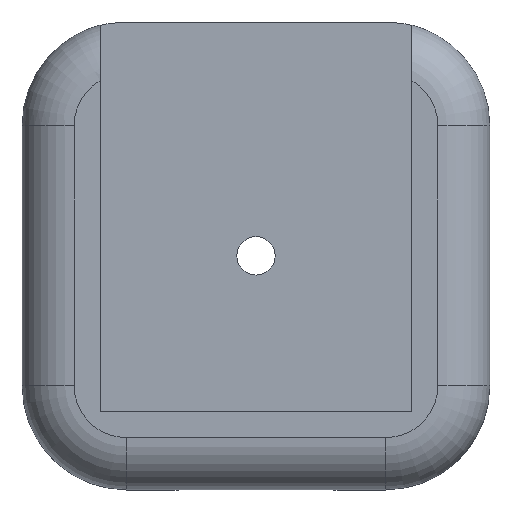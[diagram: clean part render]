
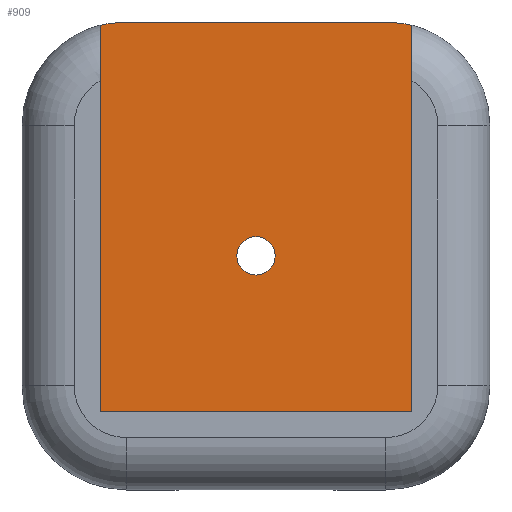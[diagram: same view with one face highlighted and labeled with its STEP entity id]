
A CAD part, top view. The second image highlights one B-rep face of the part: STEP entity #909.
In plain terms, the highlighted planar face has unit normal (0, 0, 1).
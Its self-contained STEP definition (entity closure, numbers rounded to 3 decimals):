
#11 = EDGE_CURVE ( 'NONE', #302, #878, #1433, .T. ) ;
#15 = AXIS2_PLACEMENT_3D ( 'NONE', #703, #1767, #857 ) ;
#23 = FACE_BOUND ( 'NONE', #1755, .T. ) ;
#51 = CIRCLE ( 'NONE', #916, 10. ) ;
#57 = AXIS2_PLACEMENT_3D ( 'NONE', #487, #1550, #638 ) ;
#63 = ORIENTED_EDGE ( 'NONE', *, *, #121, .T. ) ;
#78 = CIRCLE ( 'NONE', #57, 10. ) ;
#82 = ORIENTED_EDGE ( 'NONE', *, *, #1862, .T. ) ;
#83 = CIRCLE ( 'NONE', #15, 1.844 ) ;
#121 = EDGE_CURVE ( 'NONE', #176, #630, #78, .T. ) ;
#153 = DIRECTION ( 'NONE',  ( 0., 1., 0. ) ) ;
#156 = LINE ( 'NONE', #1726, #1732 ) ;
#169 = DIRECTION ( 'NONE',  ( 0., 0., 1. ) ) ;
#176 = VERTEX_POINT ( 'NONE', #191 ) ;
#187 = AXIS2_PLACEMENT_3D ( 'NONE', #1717, #808, #1872 ) ;
#191 = CARTESIAN_POINT ( 'NONE',  ( 30., 28.66, 8.75 ) ) ;
#258 = VECTOR ( 'NONE', #153, 1000. ) ;
#265 = EDGE_LOOP ( 'NONE', ( #1849, #63, #567, #1904, #395, #806 ) ) ;
#288 = VERTEX_POINT ( 'NONE', #835 ) ;
#302 = VERTEX_POINT ( 'NONE', #1449 ) ;
#319 = LINE ( 'NONE', #1265, #1488 ) ;
#377 = EDGE_CURVE ( 'NONE', #1473, #1205, #83, .T. ) ;
#395 = ORIENTED_EDGE ( 'NONE', *, *, #11, .F. ) ;
#444 = VERTEX_POINT ( 'NONE', #1170 ) ;
#487 = CARTESIAN_POINT ( 'NONE',  ( 25., 20., 8.75 ) ) ;
#567 = ORIENTED_EDGE ( 'NONE', *, *, #1934, .F. ) ;
#630 = VERTEX_POINT ( 'NONE', #1384 ) ;
#638 = DIRECTION ( 'NONE',  ( 1., 0., 0. ) ) ;
#691 = DIRECTION ( 'NONE',  ( 1., 0., 0. ) ) ;
#703 = CARTESIAN_POINT ( 'NONE',  ( 12.5, 7.5, 8.75 ) ) ;
#806 = ORIENTED_EDGE ( 'NONE', *, *, #824, .F. ) ;
#808 = DIRECTION ( 'NONE',  ( 0., 0., -1. ) ) ;
#822 = CIRCLE ( 'NONE', #187, 1.844 ) ;
#824 = EDGE_CURVE ( 'NONE', #288, #302, #1013, .T. ) ;
#835 = CARTESIAN_POINT ( 'NONE',  ( 30., -7.5, 8.75 ) ) ;
#857 = DIRECTION ( 'NONE',  ( 1., 0., 0. ) ) ;
#878 = VERTEX_POINT ( 'NONE', #1731 ) ;
#909 = ADVANCED_FACE ( 'NONE', ( #23, #1179 ), #1749, .T. ) ;
#916 = AXIS2_PLACEMENT_3D ( 'NONE', #1085, #169, #1236 ) ;
#954 = AXIS2_PLACEMENT_3D ( 'NONE', #1139, #1599, #691 ) ;
#1013 = LINE ( 'NONE', #1575, #1966 ) ;
#1065 = CARTESIAN_POINT ( 'NONE',  ( -5., -51.401, 8.75 ) ) ;
#1085 = CARTESIAN_POINT ( 'NONE',  ( 0., 20., 8.75 ) ) ;
#1139 = CARTESIAN_POINT ( 'NONE',  ( 0., -51.401, 8.75 ) ) ;
#1143 = EDGE_CURVE ( 'NONE', #444, #878, #51, .T. ) ;
#1170 = CARTESIAN_POINT ( 'NONE',  ( 0., 30., 8.75 ) ) ;
#1179 = FACE_OUTER_BOUND ( 'NONE', #265, .T. ) ;
#1205 = VERTEX_POINT ( 'NONE', #1860 ) ;
#1236 = DIRECTION ( 'NONE',  ( 1., 0., 0. ) ) ;
#1265 = CARTESIAN_POINT ( 'NONE',  ( 0., 30., 8.75 ) ) ;
#1317 = EDGE_CURVE ( 'NONE', #288, #176, #156, .T. ) ;
#1384 = CARTESIAN_POINT ( 'NONE',  ( 25., 30., 8.75 ) ) ;
#1405 = ORIENTED_EDGE ( 'NONE', *, *, #377, .T. ) ;
#1433 = LINE ( 'NONE', #1065, #258 ) ;
#1449 = CARTESIAN_POINT ( 'NONE',  ( -5., -7.5, 8.75 ) ) ;
#1473 = VERTEX_POINT ( 'NONE', #1921 ) ;
#1488 = VECTOR ( 'NONE', #1578, 1000. ) ;
#1550 = DIRECTION ( 'NONE',  ( 0., 0., 1. ) ) ;
#1567 = DIRECTION ( 'NONE',  ( -1., 0., 0. ) ) ;
#1575 = CARTESIAN_POINT ( 'NONE',  ( 0., -7.5, 8.75 ) ) ;
#1578 = DIRECTION ( 'NONE',  ( 1., 0., 0. ) ) ;
#1599 = DIRECTION ( 'NONE',  ( 0., 0., 1. ) ) ;
#1717 = CARTESIAN_POINT ( 'NONE',  ( 12.5, 7.5, 8.75 ) ) ;
#1726 = CARTESIAN_POINT ( 'NONE',  ( 30., -51.401, 8.75 ) ) ;
#1731 = CARTESIAN_POINT ( 'NONE',  ( -5., 28.66, 8.75 ) ) ;
#1732 = VECTOR ( 'NONE', #1738, 1000. ) ;
#1738 = DIRECTION ( 'NONE',  ( 0., 1., 0. ) ) ;
#1749 = PLANE ( 'NONE',  #954 ) ;
#1755 = EDGE_LOOP ( 'NONE', ( #82, #1405 ) ) ;
#1767 = DIRECTION ( 'NONE',  ( 0., 0., -1. ) ) ;
#1849 = ORIENTED_EDGE ( 'NONE', *, *, #1317, .T. ) ;
#1860 = CARTESIAN_POINT ( 'NONE',  ( 12.5, 9.344, 8.75 ) ) ;
#1862 = EDGE_CURVE ( 'NONE', #1205, #1473, #822, .T. ) ;
#1872 = DIRECTION ( 'NONE',  ( 1., 0., 0. ) ) ;
#1904 = ORIENTED_EDGE ( 'NONE', *, *, #1143, .T. ) ;
#1921 = CARTESIAN_POINT ( 'NONE',  ( 12.5, 5.656, 8.75 ) ) ;
#1934 = EDGE_CURVE ( 'NONE', #444, #630, #319, .T. ) ;
#1966 = VECTOR ( 'NONE', #1567, 1000. ) ;
